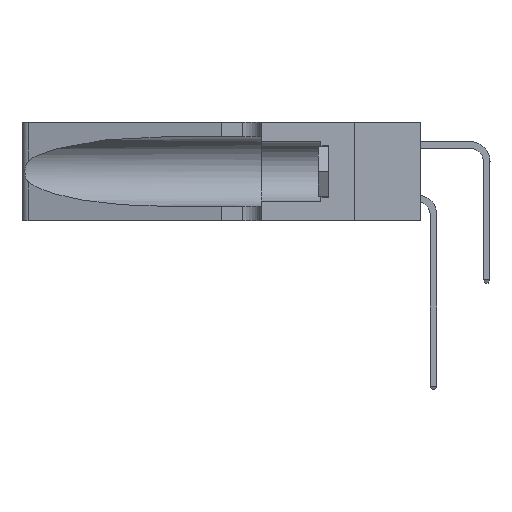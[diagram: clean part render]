
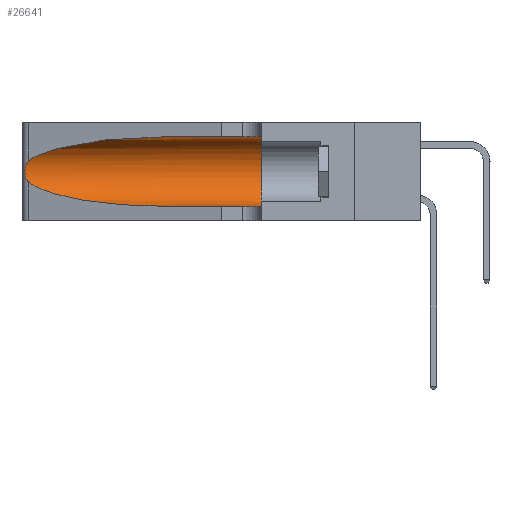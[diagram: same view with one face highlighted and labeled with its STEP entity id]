
A CAD part, left-side view. The second image highlights one B-rep face of the part: STEP entity #26641.
In plain terms, the highlighted cylindrical face has radius 3.308 mm (diameter 6.617 mm), a partial arc.
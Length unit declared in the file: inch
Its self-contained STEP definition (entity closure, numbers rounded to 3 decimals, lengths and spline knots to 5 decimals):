
#116 = CIRCLE ( 'NONE', #35973, 0.13025 ) ;
#1080 = CARTESIAN_POINT ( 'NONE',  ( 0.1305, 1.61858, 0.05475 ) ) ;
#1531 = VERTEX_POINT ( 'NONE', #19340 ) ;
#2353 = LINE ( 'NONE', #1080, #31301 ) ;
#2418 = ORIENTED_EDGE ( 'NONE', *, *, #35273, .F. ) ;
#2467 = CARTESIAN_POINT ( 'NONE',  ( 0.1305, 0.72297, 0.05475 ) ) ;
#2687 = CARTESIAN_POINT ( 'NONE',  ( 0.18966, 0.96281, 0.31525 ) ) ;
#3251 = CARTESIAN_POINT ( 'NONE',  ( 0.25487, 1.22718, 0.22369 ) ) ;
#3289 = DIRECTION ( 'NONE',  ( 0., 0., -1. ) ) ;
#4112 = DIRECTION ( 'NONE',  ( 0., -1., 0. ) ) ;
#4344 = CARTESIAN_POINT ( 'NONE',  ( 0.25787, 1.23484, 0.2124 ) ) ;
#4478 = VERTEX_POINT ( 'NONE', #3251 ) ;
#5708 = CARTESIAN_POINT ( 'NONE',  ( 0.25487, 1.22718, 0.22369 ) ) ;
#6033 = EDGE_LOOP ( 'NONE', ( #19880, #25765, #22048, #12187, #20238, #2418 ) ) ;
#7360 = CARTESIAN_POINT ( 'NONE',  ( 0.1305, 0.35, 0.185 ) ) ;
#7370 = CARTESIAN_POINT ( 'NONE',  ( 0.26018, 1.23835, 0.19895 ) ) ;
#8700 = CARTESIAN_POINT ( 'NONE',  ( 0.1305, 1.61858, 0.31525 ) ) ;
#10270 = DIRECTION ( 'NONE',  ( 0., 0., 1. ) ) ;
#10285 = CARTESIAN_POINT ( 'NONE',  ( 0.26075, 1.23896, 0.178 ) ) ;
#10485 = VERTEX_POINT ( 'NONE', #2467 ) ;
#11546 = EDGE_CURVE ( 'NONE', #10485, #13546, #2353, .T. ) ;
#11628 = CYLINDRICAL_SURFACE ( 'NONE', #16777, 0.13025 ) ;
#12187 = ORIENTED_EDGE ( 'NONE', *, *, #11546, .T. ) ;
#13200 = CARTESIAN_POINT ( 'NONE',  ( 0.25856, 1.23593, 0.16098 ) ) ;
#13546 = VERTEX_POINT ( 'NONE', #18616 ) ;
#14375 =( BOUNDED_CURVE ( )  B_SPLINE_CURVE ( 3, ( #17255, #2687, #22975, #5708 ),
 .UNSPECIFIED., .F., .T. ) 
 B_SPLINE_CURVE_WITH_KNOTS ( ( 4, 4 ),
 ( 1.5708, 2.84003 ),
 .UNSPECIFIED. ) 
 CURVE ( )  GEOMETRIC_REPRESENTATION_ITEM ( )  RATIONAL_B_SPLINE_CURVE ( ( 1., 0.87, 0.87, 1. ) ) 
 REPRESENTATION_ITEM ( '' )  );
#14540 = VECTOR ( 'NONE', #31615, 39.37008 ) ;
#14968 = CARTESIAN_POINT ( 'NONE',  ( 0.18966, 0.96281, 0.05475 ) ) ;
#15451 = LINE ( 'NONE', #8700, #14540 ) ;
#15564 = CARTESIAN_POINT ( 'NONE',  ( 0.1305, 0.72297, 0.31525 ) ) ;
#16089 = CARTESIAN_POINT ( 'NONE',  ( 0.25639, 1.23186, 0.15144 ) ) ;
#16777 = AXIS2_PLACEMENT_3D ( 'NONE', #20683, #32039, #3289 ) ;
#16785 = VERTEX_POINT ( 'NONE', #15564 ) ;
#17255 = CARTESIAN_POINT ( 'NONE',  ( 0.1305, 0.72297, 0.31525 ) ) ;
#17630 = CARTESIAN_POINT ( 'NONE',  ( 0.1305, 0.35, 0.31525 ) ) ;
#17725 = CARTESIAN_POINT ( 'NONE',  ( 0.25487, 1.22718, 0.14631 ) ) ;
#18616 = CARTESIAN_POINT ( 'NONE',  ( 0.1305, 0.35, 0.05475 ) ) ;
#18945 = CARTESIAN_POINT ( 'NONE',  ( 0.25487, 1.22718, 0.14631 ) ) ;
#19340 = CARTESIAN_POINT ( 'NONE',  ( 0.25487, 1.22718, 0.14631 ) ) ;
#19628 = EDGE_CURVE ( 'NONE', #16785, #4478, #14375, .T. ) ;
#19880 = ORIENTED_EDGE ( 'NONE', *, *, #19628, .T. ) ;
#20238 = ORIENTED_EDGE ( 'NONE', *, *, #31600, .F. ) ;
#20683 = CARTESIAN_POINT ( 'NONE',  ( 0.1305, 1.61858, 0.185 ) ) ;
#21671 = CARTESIAN_POINT ( 'NONE',  ( 0.25639, 1.23184, 0.21858 ) ) ;
#22048 = ORIENTED_EDGE ( 'NONE', *, *, #36026, .T. ) ;
#22145 =( BOUNDED_CURVE ( )  B_SPLINE_CURVE ( 3, ( #17725, #26329, #14968, #34898 ),
 .UNSPECIFIED., .F., .F. ) 
 B_SPLINE_CURVE_WITH_KNOTS ( ( 4, 4 ),
 ( 3.44316, 4.71239 ),
 .UNSPECIFIED. ) 
 CURVE ( )  GEOMETRIC_REPRESENTATION_ITEM ( )  RATIONAL_B_SPLINE_CURVE ( ( 1., 0.87, 0.87, 1. ) ) 
 REPRESENTATION_ITEM ( '' )  );
#22975 = CARTESIAN_POINT ( 'NONE',  ( 0.2373, 1.15595, 0.28018 ) ) ;
#24560 = CARTESIAN_POINT ( 'NONE',  ( 0.25854, 1.2359, 0.20912 ) ) ;
#25765 = ORIENTED_EDGE ( 'NONE', *, *, #27550, .T. ) ;
#26329 = CARTESIAN_POINT ( 'NONE',  ( 0.2373, 1.15595, 0.08982 ) ) ;
#26641 = ADVANCED_FACE ( 'NONE', ( #26841 ), #11628, .F. ) ;
#26841 = FACE_OUTER_BOUND ( 'NONE', #6033, .T. ) ;
#27415 = DIRECTION ( 'NONE',  ( 0., 1., 0. ) ) ;
#27427 = CARTESIAN_POINT ( 'NONE',  ( 0.26075, 1.23896, 0.19203 ) ) ;
#27550 = EDGE_CURVE ( 'NONE', #4478, #1531, #31530, .T. ) ;
#28688 = VERTEX_POINT ( 'NONE', #17630 ) ;
#30194 = CARTESIAN_POINT ( 'NONE',  ( 0.25487, 1.22718, 0.22369 ) ) ;
#30315 = CARTESIAN_POINT ( 'NONE',  ( 0.26017, 1.23833, 0.17102 ) ) ;
#31301 = VECTOR ( 'NONE', #4112, 39.37008 ) ;
#31530 = B_SPLINE_CURVE_WITH_KNOTS ( 'NONE', 3,
 ( #30194, #33025, #21671, #4344, #24560, #7370, #27427, #10285, #30315, #13200, #33153, #16089, #35992, #18945 ),
 .UNSPECIFIED., .F., .F.,
 ( 4, 2, 2, 2, 2, 2, 4 ),
 ( 0., 0.00027, 0.00053, 0.00107, 0.0016, 0.00187, 0.00214 ),
 .UNSPECIFIED. ) ;
#31600 = EDGE_CURVE ( 'NONE', #28688, #13546, #116, .T. ) ;
#31615 = DIRECTION ( 'NONE',  ( 0., -1., 0. ) ) ;
#32039 = DIRECTION ( 'NONE',  ( 0., -1., 0. ) ) ;
#33025 = CARTESIAN_POINT ( 'NONE',  ( 0.25555, 1.22994, 0.2215 ) ) ;
#33153 = CARTESIAN_POINT ( 'NONE',  ( 0.25789, 1.23486, 0.15765 ) ) ;
#34898 = CARTESIAN_POINT ( 'NONE',  ( 0.1305, 0.72297, 0.05475 ) ) ;
#35273 = EDGE_CURVE ( 'NONE', #16785, #28688, #15451, .T. ) ;
#35973 = AXIS2_PLACEMENT_3D ( 'NONE', #7360, #27415, #10270 ) ;
#35992 = CARTESIAN_POINT ( 'NONE',  ( 0.25555, 1.22993, 0.14849 ) ) ;
#36026 = EDGE_CURVE ( 'NONE', #1531, #10485, #22145, .T. ) ;
